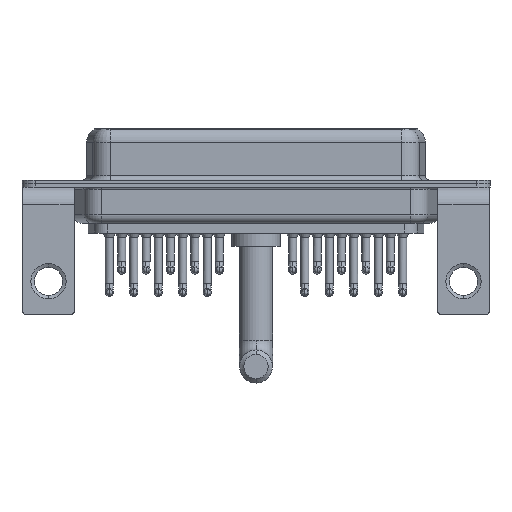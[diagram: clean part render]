
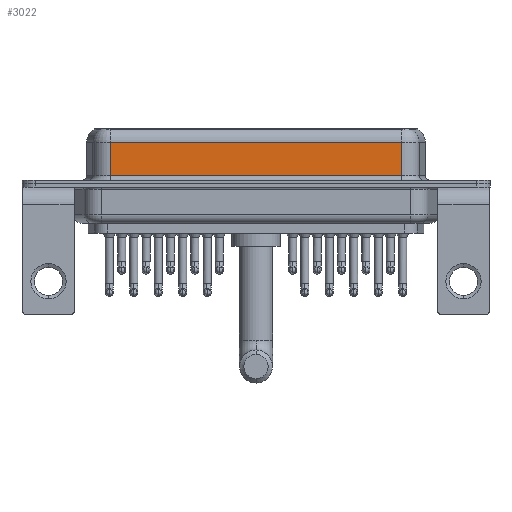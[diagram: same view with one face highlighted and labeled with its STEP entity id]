
A CAD part, front view. The second image highlights one B-rep face of the part: STEP entity #3022.
In plain terms, the highlighted planar face has unit normal (0, -1, 0).
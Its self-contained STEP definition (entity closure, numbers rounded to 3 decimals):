
#1905 = ORIENTED_EDGE ( 'NONE', *, *, #17371, .T. ) ;
#2208 = CARTESIAN_POINT ( 'NONE',  ( 7.013, -3.95, 6.4 ) ) ;
#2681 = VECTOR ( 'NONE', #3919, 1000. ) ;
#2939 = CARTESIAN_POINT ( 'NONE',  ( 40.037, -3.95, 4.65 ) ) ;
#3022 = ADVANCED_FACE ( 'NONE', ( #13596 ), #20686, .F. ) ;
#3661 = EDGE_CURVE ( 'NONE', #20913, #17410, #10786, .T. ) ;
#3919 = DIRECTION ( 'NONE',  ( 0., 0., -1. ) ) ;
#6116 = DIRECTION ( 'NONE',  ( 0., 0., -1. ) ) ;
#6230 = LINE ( 'NONE', #2208, #9531 ) ;
#6745 = LINE ( 'NONE', #2939, #17458 ) ;
#7130 = AXIS2_PLACEMENT_3D ( 'NONE', #22051, #21818, #12937 ) ;
#8329 = ORIENTED_EDGE ( 'NONE', *, *, #21002, .F. ) ;
#9531 = VECTOR ( 'NONE', #6116, 1000. ) ;
#10587 = VERTEX_POINT ( 'NONE', #11068 ) ;
#10662 = CARTESIAN_POINT ( 'NONE',  ( 40.037, -3.95, 0.9 ) ) ;
#10671 = VERTEX_POINT ( 'NONE', #13424 ) ;
#10786 = LINE ( 'NONE', #10662, #18461 ) ;
#11068 = CARTESIAN_POINT ( 'NONE',  ( 40.037, -3.95, 4.65 ) ) ;
#11376 = LINE ( 'NONE', #18575, #2681 ) ;
#12451 = CARTESIAN_POINT ( 'NONE',  ( 7.013, -3.95, 0.9 ) ) ;
#12937 = DIRECTION ( 'NONE',  ( 0., 0., 1. ) ) ;
#13424 = CARTESIAN_POINT ( 'NONE',  ( 7.013, -3.95, 4.65 ) ) ;
#13596 = FACE_OUTER_BOUND ( 'NONE', #18088, .T. ) ;
#13786 = ORIENTED_EDGE ( 'NONE', *, *, #3661, .T. ) ;
#14069 = DIRECTION ( 'NONE',  ( -1., 0., 0. ) ) ;
#17371 = EDGE_CURVE ( 'NONE', #10587, #10671, #6745, .T. ) ;
#17410 = VERTEX_POINT ( 'NONE', #21275 ) ;
#17458 = VECTOR ( 'NONE', #14069, 1000. ) ;
#17853 = DIRECTION ( 'NONE',  ( 1., 0., 0. ) ) ;
#18088 = EDGE_LOOP ( 'NONE', ( #8329, #1905, #23056, #13786 ) ) ;
#18461 = VECTOR ( 'NONE', #17853, 1000. ) ;
#18575 = CARTESIAN_POINT ( 'NONE',  ( 40.037, -3.95, 6.4 ) ) ;
#20686 = PLANE ( 'NONE',  #7130 ) ;
#20913 = VERTEX_POINT ( 'NONE', #12451 ) ;
#21002 = EDGE_CURVE ( 'NONE', #10587, #17410, #11376, .T. ) ;
#21275 = CARTESIAN_POINT ( 'NONE',  ( 40.037, -3.95, 0.9 ) ) ;
#21498 = EDGE_CURVE ( 'NONE', #10671, #20913, #6230, .T. ) ;
#21818 = DIRECTION ( 'NONE',  ( 0., 1., 0. ) ) ;
#22051 = CARTESIAN_POINT ( 'NONE',  ( 40.037, -3.95, 6.4 ) ) ;
#23056 = ORIENTED_EDGE ( 'NONE', *, *, #21498, .T. ) ;
